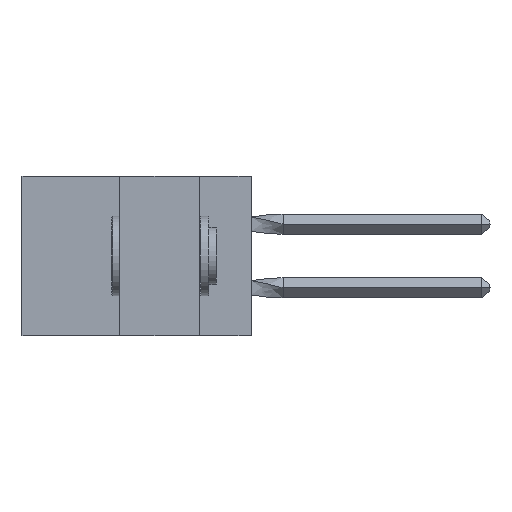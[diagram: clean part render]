
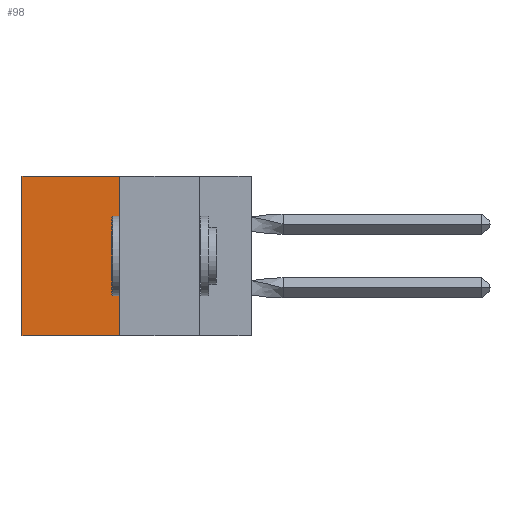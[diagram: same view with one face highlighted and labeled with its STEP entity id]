
A CAD part, left-side view. The second image highlights one B-rep face of the part: STEP entity #98.
In plain terms, the highlighted planar face has unit normal (-1, 0, 0).
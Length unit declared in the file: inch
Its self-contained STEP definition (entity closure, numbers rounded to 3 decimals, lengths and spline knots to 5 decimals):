
#98 = ADVANCED_FACE ( 'NONE', ( #3435 ), #11344, .F. ) ;
#105 = DIRECTION ( 'NONE',  ( 0., 1., 0. ) ) ;
#1526 = ORIENTED_EDGE ( 'NONE', *, *, #4143, .T. ) ;
#1618 = EDGE_LOOP ( 'NONE', ( #1526, #10249, #15377, #5088 ) ) ;
#2028 = LINE ( 'NONE', #12499, #15749 ) ;
#2095 = CARTESIAN_POINT ( 'NONE',  ( 0.305, 0.413, -0.5 ) ) ;
#3229 = CARTESIAN_POINT ( 'NONE',  ( 0.305, 0.72, -0.5 ) ) ;
#3435 = FACE_OUTER_BOUND ( 'NONE', #1618, .T. ) ;
#3495 = CARTESIAN_POINT ( 'NONE',  ( 0.305, 0.413, -0.5 ) ) ;
#4068 = DIRECTION ( 'NONE',  ( 0., 1., 0. ) ) ;
#4143 = EDGE_CURVE ( 'NONE', #6051, #16032, #9363, .T. ) ;
#4897 = LINE ( 'NONE', #10756, #10845 ) ;
#5088 = ORIENTED_EDGE ( 'NONE', *, *, #11846, .T. ) ;
#5796 = VERTEX_POINT ( 'NONE', #2095 ) ;
#6051 = VERTEX_POINT ( 'NONE', #8694 ) ;
#7368 = EDGE_CURVE ( 'NONE', #5796, #16032, #14807, .T. ) ;
#8607 = DIRECTION ( 'NONE',  ( 0., 0., -1. ) ) ;
#8694 = CARTESIAN_POINT ( 'NONE',  ( 0.305, 0.72, 0. ) ) ;
#9090 = DIRECTION ( 'NONE',  ( 0., 0., -1. ) ) ;
#9363 = LINE ( 'NONE', #16880, #14278 ) ;
#10249 = ORIENTED_EDGE ( 'NONE', *, *, #7368, .F. ) ;
#10756 = CARTESIAN_POINT ( 'NONE',  ( 0.305, 0.413, 0. ) ) ;
#10824 = AXIS2_PLACEMENT_3D ( 'NONE', #3495, #12670, #14107 ) ;
#10845 = VECTOR ( 'NONE', #4068, 39.37008 ) ;
#11344 = PLANE ( 'NONE',  #10824 ) ;
#11701 = CARTESIAN_POINT ( 'NONE',  ( 0.305, 0.413, -0.5 ) ) ;
#11846 = EDGE_CURVE ( 'NONE', #13950, #6051, #4897, .T. ) ;
#12156 = VECTOR ( 'NONE', #105, 39.37008 ) ;
#12499 = CARTESIAN_POINT ( 'NONE',  ( 0.305, 0.413, -0.5 ) ) ;
#12670 = DIRECTION ( 'NONE',  ( 1., 0., 0. ) ) ;
#13950 = VERTEX_POINT ( 'NONE', #15961 ) ;
#14107 = DIRECTION ( 'NONE',  ( 0., 0., -1. ) ) ;
#14278 = VECTOR ( 'NONE', #9090, 39.37008 ) ;
#14807 = LINE ( 'NONE', #11701, #12156 ) ;
#15377 = ORIENTED_EDGE ( 'NONE', *, *, #16763, .F. ) ;
#15749 = VECTOR ( 'NONE', #8607, 39.37008 ) ;
#15961 = CARTESIAN_POINT ( 'NONE',  ( 0.305, 0.413, 0. ) ) ;
#16032 = VERTEX_POINT ( 'NONE', #3229 ) ;
#16763 = EDGE_CURVE ( 'NONE', #13950, #5796, #2028, .T. ) ;
#16880 = CARTESIAN_POINT ( 'NONE',  ( 0.305, 0.72, -0.5 ) ) ;
